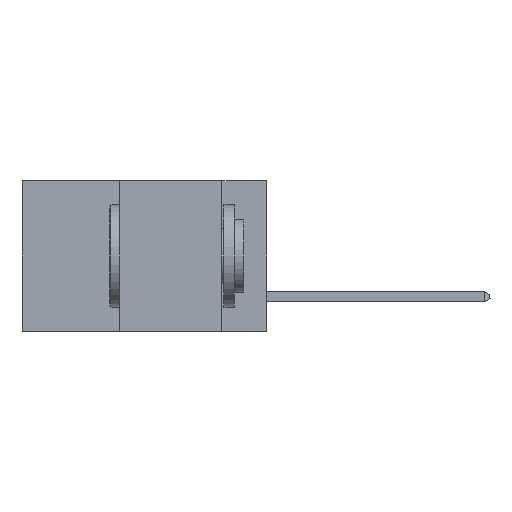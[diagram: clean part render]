
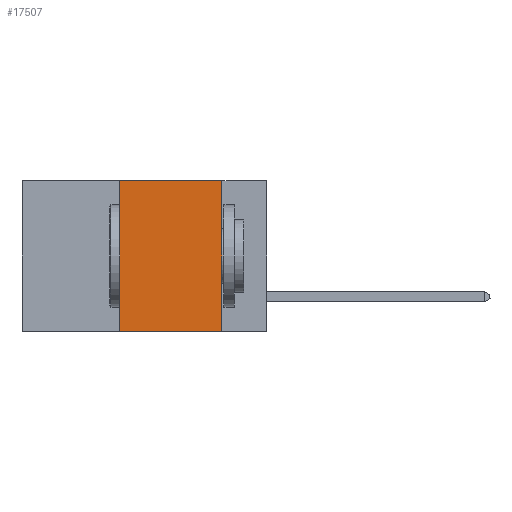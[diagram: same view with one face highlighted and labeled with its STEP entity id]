
A CAD part, left-side view. The second image highlights one B-rep face of the part: STEP entity #17507.
In plain terms, the highlighted planar face has unit normal (-1, 0, 0).
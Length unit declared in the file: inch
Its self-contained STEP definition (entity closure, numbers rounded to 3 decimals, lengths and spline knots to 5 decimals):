
#2225 = VERTEX_POINT ( 'NONE', #45177 ) ;
#4394 = CARTESIAN_POINT ( 'NONE',  ( 0., 0.6, 0. ) ) ;
#4985 = DIRECTION ( 'NONE',  ( 0., 0., -1. ) ) ;
#7027 = ORIENTED_EDGE ( 'NONE', *, *, #26100, .F. ) ;
#7692 = ORIENTED_EDGE ( 'NONE', *, *, #30139, .F. ) ;
#8095 = VECTOR ( 'NONE', #15628, 39.37008 ) ;
#8128 = FACE_OUTER_BOUND ( 'NONE', #38766, .T. ) ;
#8703 = CARTESIAN_POINT ( 'NONE',  ( 0., 0.36, -0.37 ) ) ;
#11147 = VECTOR ( 'NONE', #21394, 39.37008 ) ;
#11663 = LINE ( 'NONE', #20367, #11147 ) ;
#13766 = VERTEX_POINT ( 'NONE', #29756 ) ;
#14422 = DIRECTION ( 'NONE',  ( 0., 0., -1. ) ) ;
#15628 = DIRECTION ( 'NONE',  ( 0., -1., 0. ) ) ;
#16273 = VERTEX_POINT ( 'NONE', #8703 ) ;
#17507 = ADVANCED_FACE ( 'NONE', ( #8128 ), #27060, .F. ) ;
#19718 = AXIS2_PLACEMENT_3D ( 'NONE', #41680, #23188, #4985 ) ;
#20367 = CARTESIAN_POINT ( 'NONE',  ( 0., 0.36, 0. ) ) ;
#21394 = DIRECTION ( 'NONE',  ( 0., 0., 1. ) ) ;
#23188 = DIRECTION ( 'NONE',  ( 1., 0., 0. ) ) ;
#25103 = VECTOR ( 'NONE', #14422, 39.37008 ) ;
#25571 = ORIENTED_EDGE ( 'NONE', *, *, #46268, .F. ) ;
#25848 = EDGE_CURVE ( 'NONE', #16273, #13766, #40632, .T. ) ;
#26100 = EDGE_CURVE ( 'NONE', #2225, #41609, #44133, .T. ) ;
#27060 = PLANE ( 'NONE',  #19718 ) ;
#29575 = CARTESIAN_POINT ( 'NONE',  ( 0., 0.11, 0. ) ) ;
#29756 = CARTESIAN_POINT ( 'NONE',  ( 0., 0.11, -0.37 ) ) ;
#30139 = EDGE_CURVE ( 'NONE', #41609, #13766, #41879, .T. ) ;
#30967 = DIRECTION ( 'NONE',  ( 0., -1., 0. ) ) ;
#31143 = CARTESIAN_POINT ( 'NONE',  ( 0., 0.6, -0.37 ) ) ;
#31355 = ORIENTED_EDGE ( 'NONE', *, *, #25848, .T. ) ;
#36537 = CARTESIAN_POINT ( 'NONE',  ( 0., 0.11, 0. ) ) ;
#38766 = EDGE_LOOP ( 'NONE', ( #7692, #7027, #25571, #31355 ) ) ;
#40632 = LINE ( 'NONE', #31143, #47665 ) ;
#41609 = VERTEX_POINT ( 'NONE', #36537 ) ;
#41680 = CARTESIAN_POINT ( 'NONE',  ( 0., 0.6, 0. ) ) ;
#41879 = LINE ( 'NONE', #29575, #25103 ) ;
#44133 = LINE ( 'NONE', #4394, #8095 ) ;
#45177 = CARTESIAN_POINT ( 'NONE',  ( 0., 0.36, 0. ) ) ;
#46268 = EDGE_CURVE ( 'NONE', #16273, #2225, #11663, .T. ) ;
#47665 = VECTOR ( 'NONE', #30967, 39.37008 ) ;
